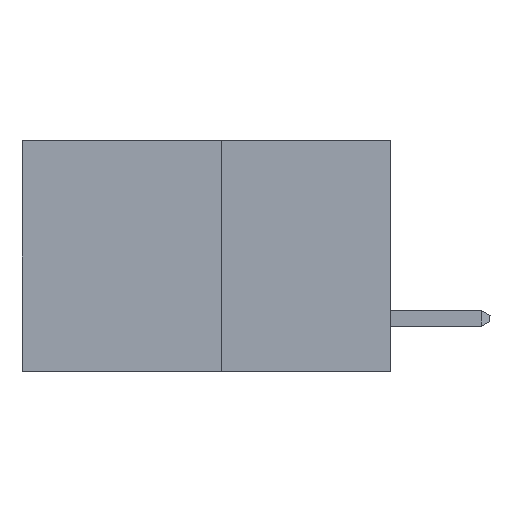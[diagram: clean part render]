
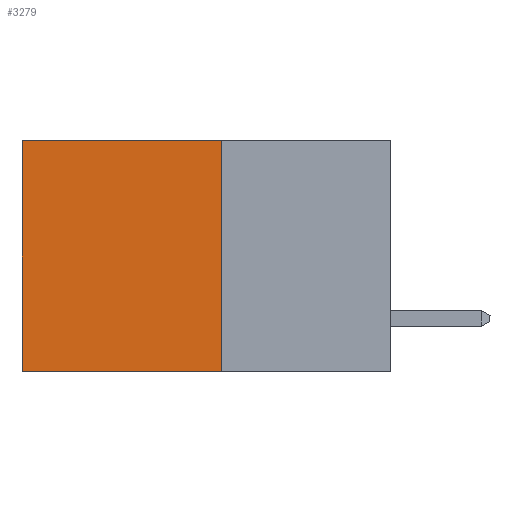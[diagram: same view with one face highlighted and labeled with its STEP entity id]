
A CAD part, left-side view. The second image highlights one B-rep face of the part: STEP entity #3279.
In plain terms, the highlighted planar face has unit normal (-1, 0, 0).
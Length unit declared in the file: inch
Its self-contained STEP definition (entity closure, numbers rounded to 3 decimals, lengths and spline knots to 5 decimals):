
#108 = CARTESIAN_POINT ( 'NONE',  ( 0.277, 0.27, 0. ) ) ;
#786 = LINE ( 'NONE', #1807, #10211 ) ;
#835 = ORIENTED_EDGE ( 'NONE', *, *, #4207, .F. ) ;
#839 = DIRECTION ( 'NONE',  ( 0., 0., -1. ) ) ;
#1317 = DIRECTION ( 'NONE',  ( 0., 0., -1. ) ) ;
#1529 = CARTESIAN_POINT ( 'NONE',  ( 0.277, 0.27, -0.37 ) ) ;
#1807 = CARTESIAN_POINT ( 'NONE',  ( 0.277, 0.59, -0.37 ) ) ;
#3025 = VERTEX_POINT ( 'NONE', #10686 ) ;
#3279 = ADVANCED_FACE ( 'NONE', ( #9274 ), #8639, .F. ) ;
#3438 = VERTEX_POINT ( 'NONE', #7492 ) ;
#4207 = EDGE_CURVE ( 'NONE', #8316, #6868, #4600, .T. ) ;
#4600 = LINE ( 'NONE', #1529, #6802 ) ;
#4940 = CARTESIAN_POINT ( 'NONE',  ( 0.277, 0.27, 0. ) ) ;
#5020 = EDGE_CURVE ( 'NONE', #3025, #3438, #786, .T. ) ;
#5074 = ORIENTED_EDGE ( 'NONE', *, *, #5020, .T. ) ;
#6341 = LINE ( 'NONE', #4940, #10921 ) ;
#6355 = LINE ( 'NONE', #10608, #10631 ) ;
#6802 = VECTOR ( 'NONE', #1317, 39.37008 ) ;
#6868 = VERTEX_POINT ( 'NONE', #8768 ) ;
#7492 = CARTESIAN_POINT ( 'NONE',  ( 0.277, 0.59, -0.37 ) ) ;
#8316 = VERTEX_POINT ( 'NONE', #108 ) ;
#8475 = ORIENTED_EDGE ( 'NONE', *, *, #10719, .T. ) ;
#8517 = DIRECTION ( 'NONE',  ( 0., 0., -1. ) ) ;
#8531 = DIRECTION ( 'NONE',  ( 1., 0., 0. ) ) ;
#8548 = CARTESIAN_POINT ( 'NONE',  ( 0.277, 0.27, -0.37 ) ) ;
#8639 = PLANE ( 'NONE',  #9886 ) ;
#8768 = CARTESIAN_POINT ( 'NONE',  ( 0.277, 0.27, -0.37 ) ) ;
#9274 = FACE_OUTER_BOUND ( 'NONE', #9852, .T. ) ;
#9852 = EDGE_LOOP ( 'NONE', ( #5074, #10537, #835, #8475 ) ) ;
#9886 = AXIS2_PLACEMENT_3D ( 'NONE', #8548, #8531, #8517 ) ;
#10211 = VECTOR ( 'NONE', #839, 39.37008 ) ;
#10316 = EDGE_CURVE ( 'NONE', #6868, #3438, #6355, .T. ) ;
#10440 = DIRECTION ( 'NONE',  ( 0., 1., 0. ) ) ;
#10537 = ORIENTED_EDGE ( 'NONE', *, *, #10316, .F. ) ;
#10608 = CARTESIAN_POINT ( 'NONE',  ( 0.277, 0.27, -0.37 ) ) ;
#10631 = VECTOR ( 'NONE', #10652, 39.37008 ) ;
#10652 = DIRECTION ( 'NONE',  ( 0., 1., 0. ) ) ;
#10686 = CARTESIAN_POINT ( 'NONE',  ( 0.277, 0.59, 0. ) ) ;
#10719 = EDGE_CURVE ( 'NONE', #8316, #3025, #6341, .T. ) ;
#10921 = VECTOR ( 'NONE', #10440, 39.37008 ) ;
